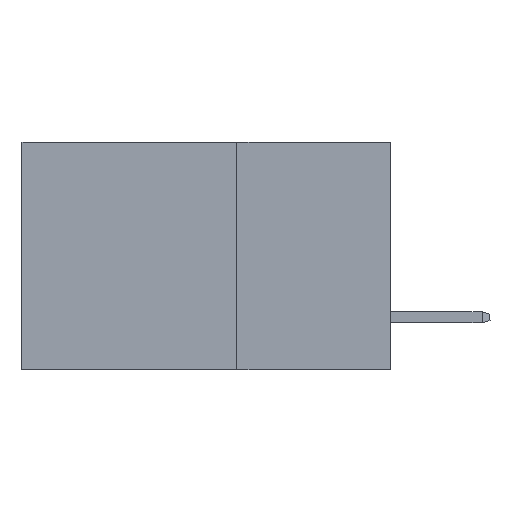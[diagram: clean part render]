
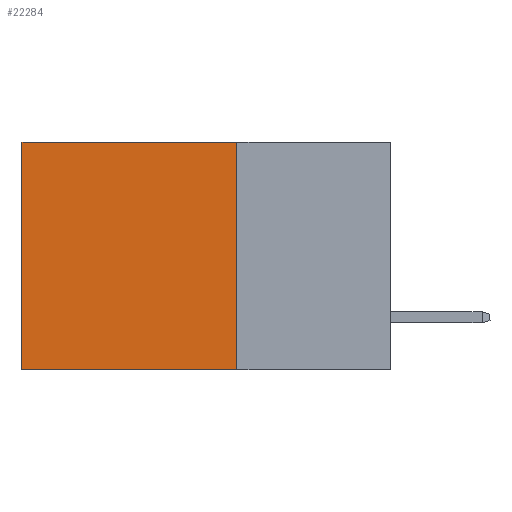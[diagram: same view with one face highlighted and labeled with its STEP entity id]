
A CAD part, left-side view. The second image highlights one B-rep face of the part: STEP entity #22284.
In plain terms, the highlighted planar face has unit normal (-1, 0, 0).
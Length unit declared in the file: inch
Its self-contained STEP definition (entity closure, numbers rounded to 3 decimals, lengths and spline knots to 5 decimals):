
#316 = CARTESIAN_POINT ( 'NONE',  ( 0.2875, 0.6, 0. ) ) ;
#644 = CARTESIAN_POINT ( 'NONE',  ( 0.2875, 0.25, 0. ) ) ;
#1217 = DIRECTION ( 'NONE',  ( 0., 0., -1. ) ) ;
#1974 = VECTOR ( 'NONE', #25265, 39.37008 ) ;
#3302 = PLANE ( 'NONE',  #23438 ) ;
#4328 = LINE ( 'NONE', #8927, #24518 ) ;
#5782 = ORIENTED_EDGE ( 'NONE', *, *, #27435, .T. ) ;
#6716 = VERTEX_POINT ( 'NONE', #18445 ) ;
#7006 = LINE ( 'NONE', #16986, #20212 ) ;
#7451 = VERTEX_POINT ( 'NONE', #316 ) ;
#8582 = DIRECTION ( 'NONE',  ( 0., 0., -1. ) ) ;
#8927 = CARTESIAN_POINT ( 'NONE',  ( 0.2875, 0.25, 0. ) ) ;
#9005 = LINE ( 'NONE', #14688, #1974 ) ;
#10471 = ORIENTED_EDGE ( 'NONE', *, *, #12073, .F. ) ;
#11557 = DIRECTION ( 'NONE',  ( 0., 0., -1. ) ) ;
#11718 = CARTESIAN_POINT ( 'NONE',  ( 0.2875, 0.6, -0.37 ) ) ;
#12073 = EDGE_CURVE ( 'NONE', #21759, #6716, #4328, .T. ) ;
#14688 = CARTESIAN_POINT ( 'NONE',  ( 0.2875, 0.25, 0. ) ) ;
#16121 = LINE ( 'NONE', #24462, #29284 ) ;
#16986 = CARTESIAN_POINT ( 'NONE',  ( 0.2875, 0.6, 0. ) ) ;
#18183 = FACE_OUTER_BOUND ( 'NONE', #29489, .T. ) ;
#18445 = CARTESIAN_POINT ( 'NONE',  ( 0.2875, 0.25, -0.37 ) ) ;
#20212 = VECTOR ( 'NONE', #1217, 39.37008 ) ;
#21759 = VERTEX_POINT ( 'NONE', #32883 ) ;
#22130 = EDGE_CURVE ( 'NONE', #6716, #28329, #16121, .T. ) ;
#22284 = ADVANCED_FACE ( 'NONE', ( #18183 ), #3302, .F. ) ;
#23438 = AXIS2_PLACEMENT_3D ( 'NONE', #644, #24346, #8582 ) ;
#23838 = EDGE_CURVE ( 'NONE', #21759, #7451, #9005, .T. ) ;
#24346 = DIRECTION ( 'NONE',  ( 1., 0., 0. ) ) ;
#24462 = CARTESIAN_POINT ( 'NONE',  ( 0.2875, 0.25, -0.37 ) ) ;
#24518 = VECTOR ( 'NONE', #11557, 39.37008 ) ;
#25265 = DIRECTION ( 'NONE',  ( 0., 1., 0. ) ) ;
#27116 = DIRECTION ( 'NONE',  ( 0., 1., 0. ) ) ;
#27435 = EDGE_CURVE ( 'NONE', #7451, #28329, #7006, .T. ) ;
#28329 = VERTEX_POINT ( 'NONE', #11718 ) ;
#28625 = ORIENTED_EDGE ( 'NONE', *, *, #23838, .T. ) ;
#29284 = VECTOR ( 'NONE', #27116, 39.37008 ) ;
#29489 = EDGE_LOOP ( 'NONE', ( #5782, #32227, #10471, #28625 ) ) ;
#32227 = ORIENTED_EDGE ( 'NONE', *, *, #22130, .F. ) ;
#32883 = CARTESIAN_POINT ( 'NONE',  ( 0.2875, 0.25, 0. ) ) ;
